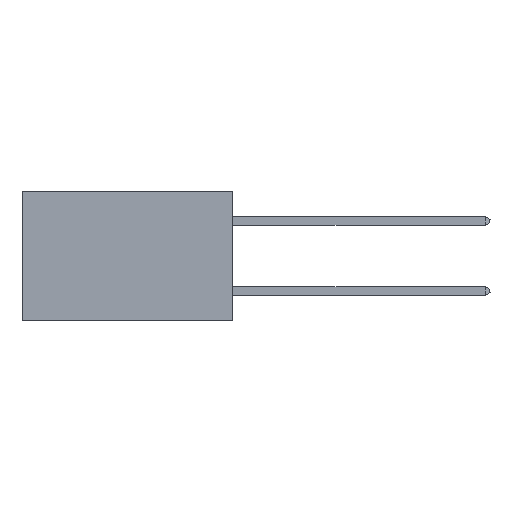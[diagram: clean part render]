
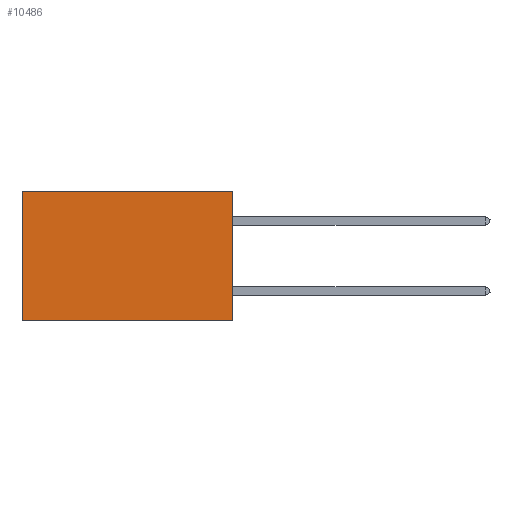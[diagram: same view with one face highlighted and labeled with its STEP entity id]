
A CAD part, left-side view. The second image highlights one B-rep face of the part: STEP entity #10486.
In plain terms, the highlighted planar face has unit normal (-1, 0, 0).
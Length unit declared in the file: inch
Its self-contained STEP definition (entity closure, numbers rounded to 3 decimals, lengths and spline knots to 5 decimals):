
#106 = VERTEX_POINT ( 'NONE', #8991 ) ;
#1080 = DIRECTION ( 'NONE',  ( 0., 0., -1. ) ) ;
#1256 = LINE ( 'NONE', #16821, #3140 ) ;
#1409 = CARTESIAN_POINT ( 'NONE',  ( 0.2875, 0., -0.37 ) ) ;
#1540 = DIRECTION ( 'NONE',  ( 0., 0., -1. ) ) ;
#2418 = CARTESIAN_POINT ( 'NONE',  ( 0.2875, 0.6, 0. ) ) ;
#3140 = VECTOR ( 'NONE', #26153, 39.37008 ) ;
#4230 = DIRECTION ( 'NONE',  ( 0., 1., 0. ) ) ;
#7222 = EDGE_LOOP ( 'NONE', ( #23816, #35506, #36087, #30592 ) ) ;
#8112 = CARTESIAN_POINT ( 'NONE',  ( 0.2875, 0.6, 0. ) ) ;
#8885 = DIRECTION ( 'NONE',  ( 0., 0., -1. ) ) ;
#8991 = CARTESIAN_POINT ( 'NONE',  ( 0.2875, 0., 0. ) ) ;
#10188 = VERTEX_POINT ( 'NONE', #37501 ) ;
#10369 = LINE ( 'NONE', #1409, #17448 ) ;
#10486 = ADVANCED_FACE ( 'NONE', ( #22030 ), #38526, .F. ) ;
#11563 = EDGE_CURVE ( 'NONE', #106, #38800, #1256, .T. ) ;
#12260 = CARTESIAN_POINT ( 'NONE',  ( 0.2875, 0.6, -0.37 ) ) ;
#16821 = CARTESIAN_POINT ( 'NONE',  ( 0.2875, 0., 0. ) ) ;
#17448 = VECTOR ( 'NONE', #4230, 39.37008 ) ;
#17608 = EDGE_CURVE ( 'NONE', #10188, #18149, #10369, .T. ) ;
#18149 = VERTEX_POINT ( 'NONE', #12260 ) ;
#18395 = EDGE_CURVE ( 'NONE', #38800, #18149, #31038, .T. ) ;
#19112 = CARTESIAN_POINT ( 'NONE',  ( 0.2875, 0., 0. ) ) ;
#20735 = CARTESIAN_POINT ( 'NONE',  ( 0.2875, 0., 0. ) ) ;
#22030 = FACE_OUTER_BOUND ( 'NONE', #7222, .T. ) ;
#23816 = ORIENTED_EDGE ( 'NONE', *, *, #18395, .T. ) ;
#26153 = DIRECTION ( 'NONE',  ( 0., 1., 0. ) ) ;
#26164 = EDGE_CURVE ( 'NONE', #106, #10188, #37469, .T. ) ;
#28440 = AXIS2_PLACEMENT_3D ( 'NONE', #20735, #35873, #8885 ) ;
#29146 = VECTOR ( 'NONE', #1540, 39.37008 ) ;
#30592 = ORIENTED_EDGE ( 'NONE', *, *, #11563, .T. ) ;
#31038 = LINE ( 'NONE', #8112, #29146 ) ;
#32279 = VECTOR ( 'NONE', #1080, 39.37008 ) ;
#35506 = ORIENTED_EDGE ( 'NONE', *, *, #17608, .F. ) ;
#35873 = DIRECTION ( 'NONE',  ( 1., 0., 0. ) ) ;
#36087 = ORIENTED_EDGE ( 'NONE', *, *, #26164, .F. ) ;
#37469 = LINE ( 'NONE', #19112, #32279 ) ;
#37501 = CARTESIAN_POINT ( 'NONE',  ( 0.2875, 0., -0.37 ) ) ;
#38526 = PLANE ( 'NONE',  #28440 ) ;
#38800 = VERTEX_POINT ( 'NONE', #2418 ) ;
